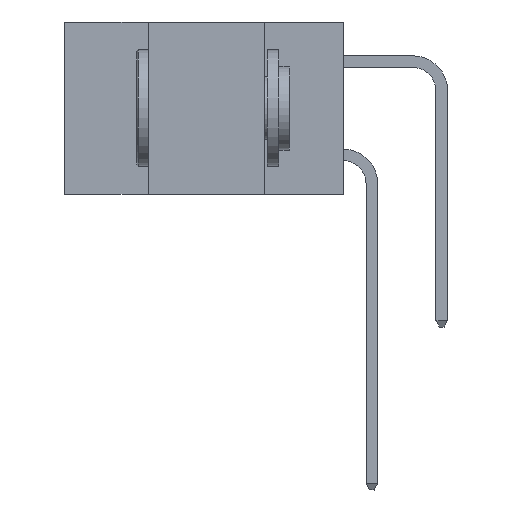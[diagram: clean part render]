
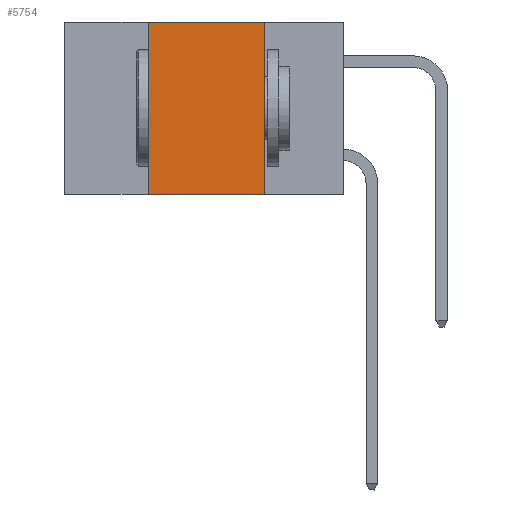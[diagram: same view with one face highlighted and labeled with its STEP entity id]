
A CAD part, left-side view. The second image highlights one B-rep face of the part: STEP entity #5754.
In plain terms, the highlighted planar face has unit normal (-1, 0, 0).
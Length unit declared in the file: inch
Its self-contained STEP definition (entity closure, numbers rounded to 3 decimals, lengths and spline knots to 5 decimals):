
#390 = CARTESIAN_POINT ( 'NONE',  ( 0., 0.17, 0. ) ) ;
#482 = VERTEX_POINT ( 'NONE', #14353 ) ;
#651 = DIRECTION ( 'NONE',  ( 0., 0., 1. ) ) ;
#1145 = EDGE_LOOP ( 'NONE', ( #19992, #1735, #7048, #12324 ) ) ;
#1504 = VERTEX_POINT ( 'NONE', #9534 ) ;
#1682 = FACE_OUTER_BOUND ( 'NONE', #1145, .T. ) ;
#1735 = ORIENTED_EDGE ( 'NONE', *, *, #15338, .F. ) ;
#4967 = CARTESIAN_POINT ( 'NONE',  ( 0., 0.6, -0.37 ) ) ;
#5754 = ADVANCED_FACE ( 'NONE', ( #1682 ), #18996, .F. ) ;
#5821 = VECTOR ( 'NONE', #20830, 39.37008 ) ;
#7048 = ORIENTED_EDGE ( 'NONE', *, *, #8240, .F. ) ;
#7171 = VECTOR ( 'NONE', #651, 39.37008 ) ;
#8003 = CARTESIAN_POINT ( 'NONE',  ( 0., 0.17, -0.37 ) ) ;
#8240 = EDGE_CURVE ( 'NONE', #8742, #482, #20657, .T. ) ;
#8456 = DIRECTION ( 'NONE',  ( 1., 0., 0. ) ) ;
#8742 = VERTEX_POINT ( 'NONE', #14681 ) ;
#9430 = EDGE_CURVE ( 'NONE', #1504, #12196, #10462, .T. ) ;
#9534 = CARTESIAN_POINT ( 'NONE',  ( 0., 0.17, 0. ) ) ;
#9657 = LINE ( 'NONE', #13648, #18459 ) ;
#9891 = VECTOR ( 'NONE', #12941, 39.37008 ) ;
#10462 = LINE ( 'NONE', #390, #9891 ) ;
#10563 = LINE ( 'NONE', #4967, #5821 ) ;
#11361 = CARTESIAN_POINT ( 'NONE',  ( 0., 0.42, 0. ) ) ;
#12196 = VERTEX_POINT ( 'NONE', #8003 ) ;
#12324 = ORIENTED_EDGE ( 'NONE', *, *, #14218, .T. ) ;
#12941 = DIRECTION ( 'NONE',  ( 0., 0., -1. ) ) ;
#13648 = CARTESIAN_POINT ( 'NONE',  ( 0., 0.6, 0. ) ) ;
#14218 = EDGE_CURVE ( 'NONE', #8742, #12196, #10563, .T. ) ;
#14353 = CARTESIAN_POINT ( 'NONE',  ( 0., 0.42, 0. ) ) ;
#14681 = CARTESIAN_POINT ( 'NONE',  ( 0., 0.42, -0.37 ) ) ;
#15338 = EDGE_CURVE ( 'NONE', #482, #1504, #9657, .T. ) ;
#15627 = AXIS2_PLACEMENT_3D ( 'NONE', #20666, #8456, #20743 ) ;
#18459 = VECTOR ( 'NONE', #22308, 39.37008 ) ;
#18996 = PLANE ( 'NONE',  #15627 ) ;
#19992 = ORIENTED_EDGE ( 'NONE', *, *, #9430, .F. ) ;
#20657 = LINE ( 'NONE', #11361, #7171 ) ;
#20666 = CARTESIAN_POINT ( 'NONE',  ( 0., 0.6, 0. ) ) ;
#20743 = DIRECTION ( 'NONE',  ( 0., 0., -1. ) ) ;
#20830 = DIRECTION ( 'NONE',  ( 0., -1., 0. ) ) ;
#22308 = DIRECTION ( 'NONE',  ( 0., -1., 0. ) ) ;
